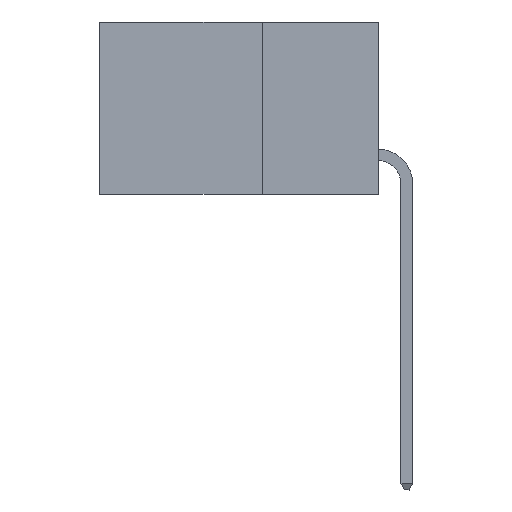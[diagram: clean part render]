
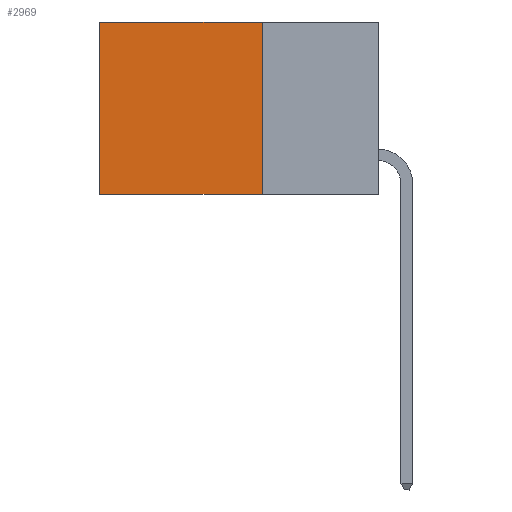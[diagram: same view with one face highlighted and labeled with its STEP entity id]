
A CAD part, left-side view. The second image highlights one B-rep face of the part: STEP entity #2969.
In plain terms, the highlighted planar face has unit normal (-1, 0, 0).
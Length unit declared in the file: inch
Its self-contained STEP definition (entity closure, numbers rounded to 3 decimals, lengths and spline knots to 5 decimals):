
#487 = VECTOR ( 'NONE', #4372, 39.37008 ) ;
#1039 = VECTOR ( 'NONE', #5421, 39.37008 ) ;
#1113 = EDGE_LOOP ( 'NONE', ( #3453, #5673, #1694, #1242 ) ) ;
#1117 = EDGE_CURVE ( 'NONE', #3059, #4802, #6653, .T. ) ;
#1242 = ORIENTED_EDGE ( 'NONE', *, *, #5073, .T. ) ;
#1277 = LINE ( 'NONE', #4615, #1039 ) ;
#1373 = CARTESIAN_POINT ( 'NONE',  ( 0.298, 0.25, 0. ) ) ;
#1521 = EDGE_CURVE ( 'NONE', #4640, #7686, #9929, .T. ) ;
#1694 = ORIENTED_EDGE ( 'NONE', *, *, #1117, .F. ) ;
#1778 = LINE ( 'NONE', #5610, #3936 ) ;
#1807 = CARTESIAN_POINT ( 'NONE',  ( 0.298, 0.25, -0.37 ) ) ;
#2069 = PLANE ( 'NONE',  #6697 ) ;
#2969 = ADVANCED_FACE ( 'NONE', ( #8398 ), #2069, .F. ) ;
#3059 = VERTEX_POINT ( 'NONE', #1373 ) ;
#3235 = CARTESIAN_POINT ( 'NONE',  ( 0.298, 0.6, -0.37 ) ) ;
#3453 = ORIENTED_EDGE ( 'NONE', *, *, #1521, .T. ) ;
#3704 = DIRECTION ( 'NONE',  ( 1., 0., 0. ) ) ;
#3936 = VECTOR ( 'NONE', #5561, 39.37008 ) ;
#4372 = DIRECTION ( 'NONE',  ( 0., 0., -1. ) ) ;
#4578 = EDGE_CURVE ( 'NONE', #4802, #7686, #1778, .T. ) ;
#4615 = CARTESIAN_POINT ( 'NONE',  ( 0.298, 0.25, 0. ) ) ;
#4640 = VERTEX_POINT ( 'NONE', #9684 ) ;
#4802 = VERTEX_POINT ( 'NONE', #1807 ) ;
#5073 = EDGE_CURVE ( 'NONE', #3059, #4640, #1277, .T. ) ;
#5421 = DIRECTION ( 'NONE',  ( 0., 1., 0. ) ) ;
#5561 = DIRECTION ( 'NONE',  ( 0., 1., 0. ) ) ;
#5610 = CARTESIAN_POINT ( 'NONE',  ( 0.298, 0.25, -0.37 ) ) ;
#5673 = ORIENTED_EDGE ( 'NONE', *, *, #4578, .F. ) ;
#6653 = LINE ( 'NONE', #9208, #487 ) ;
#6697 = AXIS2_PLACEMENT_3D ( 'NONE', #8557, #3704, #9358 ) ;
#7686 = VERTEX_POINT ( 'NONE', #3235 ) ;
#8212 = CARTESIAN_POINT ( 'NONE',  ( 0.298, 0.6, 0. ) ) ;
#8398 = FACE_OUTER_BOUND ( 'NONE', #1113, .T. ) ;
#8557 = CARTESIAN_POINT ( 'NONE',  ( 0.298, 0.25, 0. ) ) ;
#9035 = DIRECTION ( 'NONE',  ( 0., 0., -1. ) ) ;
#9208 = CARTESIAN_POINT ( 'NONE',  ( 0.298, 0.25, 0. ) ) ;
#9358 = DIRECTION ( 'NONE',  ( 0., 0., -1. ) ) ;
#9434 = VECTOR ( 'NONE', #9035, 39.37008 ) ;
#9684 = CARTESIAN_POINT ( 'NONE',  ( 0.298, 0.6, 0. ) ) ;
#9929 = LINE ( 'NONE', #8212, #9434 ) ;
